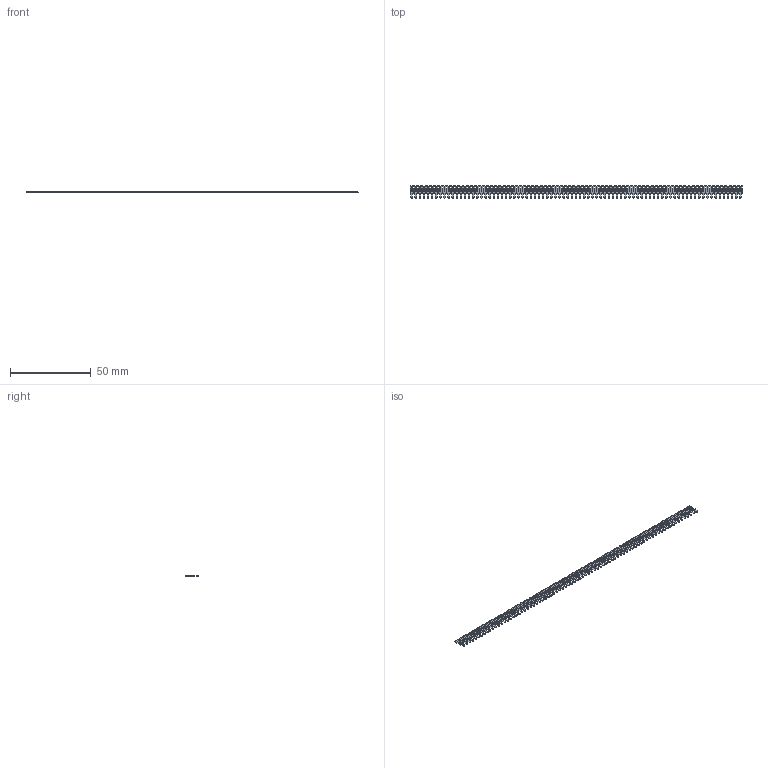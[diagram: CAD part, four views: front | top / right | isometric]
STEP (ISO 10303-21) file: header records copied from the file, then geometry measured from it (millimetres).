
FILE_DESCRIPTION (( 'STEP AP203' ), '1' );
FILE_NAME ('103-081-253-100.STEP', '2020-04-16T16:54:17', ( '' ), ( '' ), 'SwSTEP 2.0', 'SolidWorks 2016', '' );
FILE_SCHEMA (( 'CONFIG_CONTROL_DESIGN' ));
Length unit declared in the file: inch
Products named in the file (2): 100-290-001_100-290-253; 103-081-253-100
Assembly tree (81 placements, depth 2):
  103-081-253-100
    100-290-001_100-290-253  x81
Bounding box: 205.23 x 7.62 x 0.51 mm (x, y, z)
Volume: 446.9 mm3; surface area: 2787 mm2
Topology: 81 solids, 81 shells, 1620 faces, 4374 edges, 2916 vertices
Faces by surface type: plane 1539, cylinder 81
Entity records: 3380 total; most frequent: DIRECTION 264, CARTESIAN_POINT 194, COORDINATED_UNIVERSAL_TIME_OFFSET 172, LOCAL_TIME 172, DATE_AND_TIME 172, CALENDAR_DATE 172, ORIENTED_EDGE 108, AXIS2_PLACEMENT_3D 106
